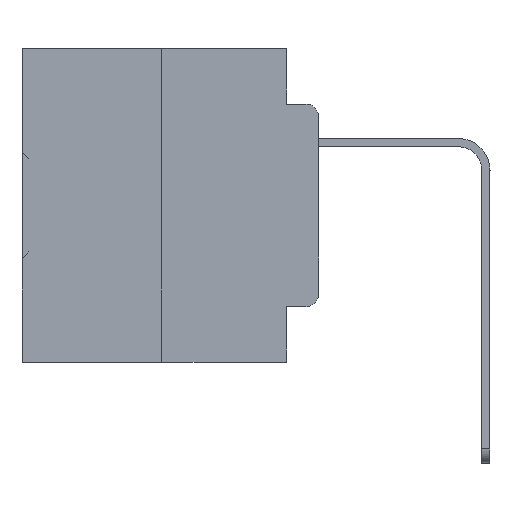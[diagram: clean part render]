
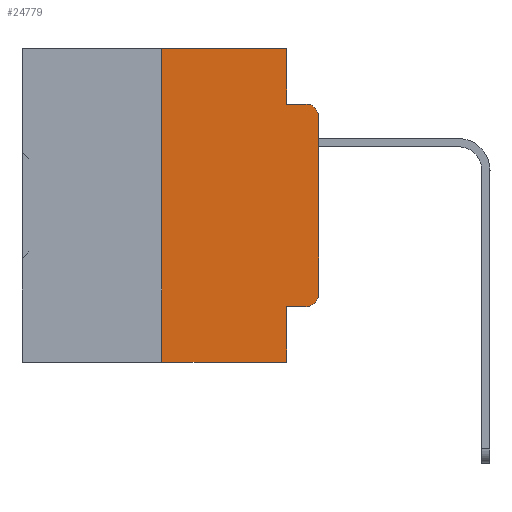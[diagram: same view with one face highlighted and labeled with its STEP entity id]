
A CAD part, left-side view. The second image highlights one B-rep face of the part: STEP entity #24779.
In plain terms, the highlighted planar face has unit normal (-1, 0, 0).
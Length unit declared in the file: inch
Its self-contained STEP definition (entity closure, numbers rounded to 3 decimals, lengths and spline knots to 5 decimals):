
#14 = LINE ( 'NONE', #10859, #30760 ) ;
#27 = CARTESIAN_POINT ( 'NONE',  ( 0., 0.02, -0.1085 ) ) ;
#356 = CARTESIAN_POINT ( 'NONE',  ( 0., 0.051, -0.4115 ) ) ;
#618 = CARTESIAN_POINT ( 'NONE',  ( 0., 0.051, -0.0885 ) ) ;
#1442 = DIRECTION ( 'NONE',  ( 0., 0., 1. ) ) ;
#1601 = CARTESIAN_POINT ( 'NONE',  ( 0., 0.02, -0.4115 ) ) ;
#1644 = VERTEX_POINT ( 'NONE', #23813 ) ;
#1894 = EDGE_CURVE ( 'NONE', #4863, #27136, #10878, .T. ) ;
#2653 = ORIENTED_EDGE ( 'NONE', *, *, #13213, .T. ) ;
#3430 = VERTEX_POINT ( 'NONE', #618 ) ;
#3695 = CARTESIAN_POINT ( 'NONE',  ( 0., 0.02, -0.3915 ) ) ;
#3951 = VERTEX_POINT ( 'NONE', #7602 ) ;
#4588 = CARTESIAN_POINT ( 'NONE',  ( 0., 0.473, 0. ) ) ;
#4610 = LINE ( 'NONE', #20328, #26443 ) ;
#4762 = DIRECTION ( 'NONE',  ( 0., 0., -1. ) ) ;
#4863 = VERTEX_POINT ( 'NONE', #356 ) ;
#5138 = VECTOR ( 'NONE', #30354, 39.37008 ) ;
#7602 = CARTESIAN_POINT ( 'NONE',  ( 0., 0.25, -0.5 ) ) ;
#9038 = VERTEX_POINT ( 'NONE', #35413 ) ;
#9040 = VERTEX_POINT ( 'NONE', #1601 ) ;
#9208 = EDGE_CURVE ( 'NONE', #3430, #13431, #11146, .T. ) ;
#9365 = EDGE_CURVE ( 'NONE', #4863, #9040, #14, .T. ) ;
#9921 = EDGE_CURVE ( 'NONE', #1644, #13431, #27632, .T. ) ;
#10625 = DIRECTION ( 'NONE',  ( 0., 0., -1. ) ) ;
#10687 = ORIENTED_EDGE ( 'NONE', *, *, #9365, .T. ) ;
#10859 = CARTESIAN_POINT ( 'NONE',  ( 0., 0.051, -0.4115 ) ) ;
#10878 = LINE ( 'NONE', #33610, #36271 ) ;
#11146 = LINE ( 'NONE', #30329, #35197 ) ;
#12577 = DIRECTION ( 'NONE',  ( 0., 0., 1. ) ) ;
#12720 = EDGE_CURVE ( 'NONE', #9038, #3430, #33137, .T. ) ;
#12788 = DIRECTION ( 'NONE',  ( 1., 0., 0. ) ) ;
#13159 = CARTESIAN_POINT ( 'NONE',  ( 0., 0.473, 0. ) ) ;
#13213 = EDGE_CURVE ( 'NONE', #3951, #27136, #26899, .T. ) ;
#13425 = ORIENTED_EDGE ( 'NONE', *, *, #27156, .T. ) ;
#13431 = VERTEX_POINT ( 'NONE', #25170 ) ;
#15374 = ORIENTED_EDGE ( 'NONE', *, *, #9208, .F. ) ;
#15758 = ORIENTED_EDGE ( 'NONE', *, *, #12720, .F. ) ;
#16250 = CIRCLE ( 'NONE', #21034, 0.02 ) ;
#16689 = VECTOR ( 'NONE', #1442, 39.37008 ) ;
#18249 = DIRECTION ( 'NONE',  ( -1., 0., 0. ) ) ;
#18952 = ORIENTED_EDGE ( 'NONE', *, *, #36131, .F. ) ;
#19309 = VECTOR ( 'NONE', #32669, 39.37008 ) ;
#19334 = ORIENTED_EDGE ( 'NONE', *, *, #27049, .T. ) ;
#19814 = DIRECTION ( 'NONE',  ( -1., 0., 0. ) ) ;
#20328 = CARTESIAN_POINT ( 'NONE',  ( 0., 0.25, 0. ) ) ;
#21034 = AXIS2_PLACEMENT_3D ( 'NONE', #3695, #18249, #23594 ) ;
#21179 = LINE ( 'NONE', #13159, #5138 ) ;
#23594 = DIRECTION ( 'NONE',  ( 0., 0., -1. ) ) ;
#23790 = CARTESIAN_POINT ( 'NONE',  ( 0., 0.25, 0. ) ) ;
#23813 = CARTESIAN_POINT ( 'NONE',  ( 0., 0., -0.1085 ) ) ;
#24003 = PLANE ( 'NONE',  #36852 ) ;
#24380 = DIRECTION ( 'NONE',  ( 0., 0., -1. ) ) ;
#24570 = CARTESIAN_POINT ( 'NONE',  ( 0., 0., 0. ) ) ;
#24779 = ADVANCED_FACE ( 'NONE', ( #31099 ), #24003, .F. ) ;
#25170 = CARTESIAN_POINT ( 'NONE',  ( 0., 0.02, -0.0885 ) ) ;
#25200 = ORIENTED_EDGE ( 'NONE', *, *, #1894, .F. ) ;
#26443 = VECTOR ( 'NONE', #12577, 39.37008 ) ;
#26899 = LINE ( 'NONE', #35741, #19309 ) ;
#26902 = ORIENTED_EDGE ( 'NONE', *, *, #9921, .T. ) ;
#27049 = EDGE_CURVE ( 'NONE', #9040, #27181, #16250, .T. ) ;
#27136 = VERTEX_POINT ( 'NONE', #35985 ) ;
#27156 = EDGE_CURVE ( 'NONE', #27181, #1644, #35792, .T. ) ;
#27181 = VERTEX_POINT ( 'NONE', #35512 ) ;
#27632 = CIRCLE ( 'NONE', #29020, 0.02 ) ;
#29020 = AXIS2_PLACEMENT_3D ( 'NONE', #27, #19814, #31379 ) ;
#30329 = CARTESIAN_POINT ( 'NONE',  ( 0., 0.051, -0.0885 ) ) ;
#30354 = DIRECTION ( 'NONE',  ( 0., -1., 0. ) ) ;
#30760 = VECTOR ( 'NONE', #31061, 39.37008 ) ;
#31061 = DIRECTION ( 'NONE',  ( 0., -1., 0. ) ) ;
#31099 = FACE_OUTER_BOUND ( 'NONE', #31787, .T. ) ;
#31379 = DIRECTION ( 'NONE',  ( 0., 0., -1. ) ) ;
#31476 = VERTEX_POINT ( 'NONE', #23790 ) ;
#31787 = EDGE_LOOP ( 'NONE', ( #13425, #26902, #15374, #15758, #36807, #18952, #2653, #25200, #10687, #19334 ) ) ;
#32669 = DIRECTION ( 'NONE',  ( 0., -1., 0. ) ) ;
#33137 = LINE ( 'NONE', #33539, #33563 ) ;
#33539 = CARTESIAN_POINT ( 'NONE',  ( 0., 0.051, 0. ) ) ;
#33563 = VECTOR ( 'NONE', #10625, 39.37008 ) ;
#33610 = CARTESIAN_POINT ( 'NONE',  ( 0., 0.051, 0. ) ) ;
#35126 = EDGE_CURVE ( 'NONE', #31476, #9038, #21179, .T. ) ;
#35197 = VECTOR ( 'NONE', #35881, 39.37008 ) ;
#35413 = CARTESIAN_POINT ( 'NONE',  ( 0., 0.051, 0. ) ) ;
#35512 = CARTESIAN_POINT ( 'NONE',  ( 0., 0., -0.3915 ) ) ;
#35741 = CARTESIAN_POINT ( 'NONE',  ( 0., 0.473, -0.5 ) ) ;
#35792 = LINE ( 'NONE', #24570, #16689 ) ;
#35881 = DIRECTION ( 'NONE',  ( 0., -1., 0. ) ) ;
#35985 = CARTESIAN_POINT ( 'NONE',  ( 0., 0.051, -0.5 ) ) ;
#36131 = EDGE_CURVE ( 'NONE', #3951, #31476, #4610, .T. ) ;
#36271 = VECTOR ( 'NONE', #4762, 39.37008 ) ;
#36807 = ORIENTED_EDGE ( 'NONE', *, *, #35126, .F. ) ;
#36852 = AXIS2_PLACEMENT_3D ( 'NONE', #4588, #12788, #24380 ) ;
